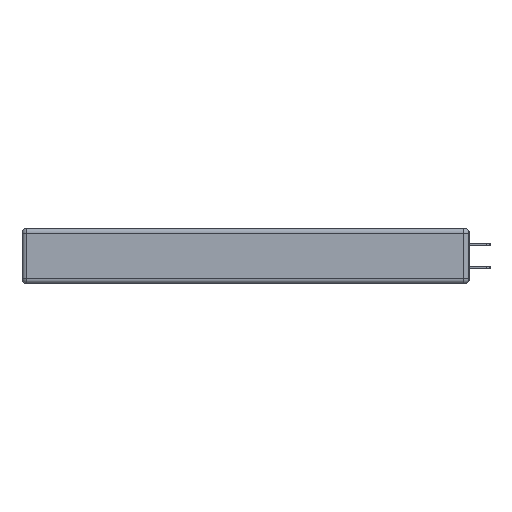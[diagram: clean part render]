
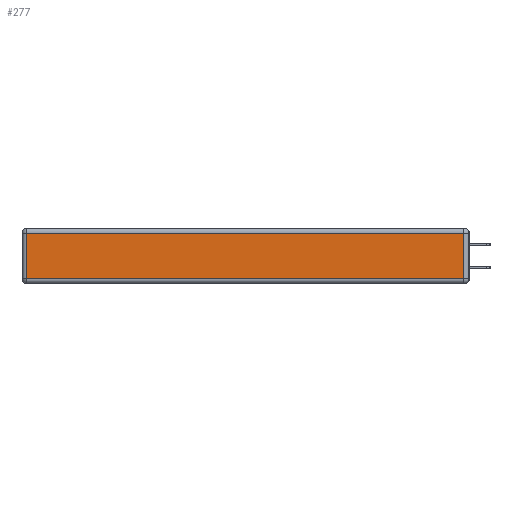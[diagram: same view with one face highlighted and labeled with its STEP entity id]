
A CAD part, left-side view. The second image highlights one B-rep face of the part: STEP entity #277.
In plain terms, the highlighted planar face has unit normal (-1, 0, 0).
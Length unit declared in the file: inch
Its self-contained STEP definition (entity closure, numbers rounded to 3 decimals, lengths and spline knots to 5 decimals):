
#159 = ORIENTED_EDGE ( 'NONE', *, *, #12862, .T. ) ;
#277 = ADVANCED_FACE ( 'NONE', ( #6587 ), #22933, .T. ) ;
#910 = CARTESIAN_POINT ( 'NONE',  ( 0., 0., -0.313 ) ) ;
#964 = VERTEX_POINT ( 'NONE', #26916 ) ;
#1173 = CARTESIAN_POINT ( 'NONE',  ( 0., 0.03, -0.313 ) ) ;
#3759 = DIRECTION ( 'NONE',  ( 0., 1., 0. ) ) ;
#4067 = DIRECTION ( 'NONE',  ( -1., 0., 0. ) ) ;
#4335 = DIRECTION ( 'NONE',  ( 0., 0., 1. ) ) ;
#6587 = FACE_OUTER_BOUND ( 'NONE', #15515, .T. ) ;
#6824 = ORIENTED_EDGE ( 'NONE', *, *, #15740, .T. ) ;
#7774 = LINE ( 'NONE', #7867, #15667 ) ;
#7867 = CARTESIAN_POINT ( 'NONE',  ( 0., 2.75, -0.03 ) ) ;
#8968 = CARTESIAN_POINT ( 'NONE',  ( 0., 2.72, -0.343 ) ) ;
#9300 = ORIENTED_EDGE ( 'NONE', *, *, #17796, .T. ) ;
#12862 = EDGE_CURVE ( 'NONE', #22538, #964, #18103, .T. ) ;
#14805 = CARTESIAN_POINT ( 'NONE',  ( 0., 0.03, -0.343 ) ) ;
#15221 = LINE ( 'NONE', #910, #18449 ) ;
#15515 = EDGE_LOOP ( 'NONE', ( #9300, #159, #6824, #23029 ) ) ;
#15667 = VECTOR ( 'NONE', #3759, 39.37008 ) ;
#15740 = EDGE_CURVE ( 'NONE', #964, #25596, #7774, .T. ) ;
#15995 = CARTESIAN_POINT ( 'NONE',  ( 0., 2.72, -0.03 ) ) ;
#17796 = EDGE_CURVE ( 'NONE', #23137, #22538, #15221, .T. ) ;
#18103 = LINE ( 'NONE', #14805, #22332 ) ;
#18449 = VECTOR ( 'NONE', #23837, 39.37008 ) ;
#18556 = CARTESIAN_POINT ( 'NONE',  ( 0., 0., -0.343 ) ) ;
#18739 = DIRECTION ( 'NONE',  ( 0., 0., 1. ) ) ;
#18831 = VECTOR ( 'NONE', #21544, 39.37008 ) ;
#21544 = DIRECTION ( 'NONE',  ( 0., 0., -1. ) ) ;
#22294 = CARTESIAN_POINT ( 'NONE',  ( 0., 2.72, -0.313 ) ) ;
#22332 = VECTOR ( 'NONE', #4335, 39.37008 ) ;
#22538 = VERTEX_POINT ( 'NONE', #1173 ) ;
#22933 = PLANE ( 'NONE',  #25558 ) ;
#23029 = ORIENTED_EDGE ( 'NONE', *, *, #25000, .T. ) ;
#23137 = VERTEX_POINT ( 'NONE', #22294 ) ;
#23714 = LINE ( 'NONE', #8968, #18831 ) ;
#23837 = DIRECTION ( 'NONE',  ( 0., -1., 0. ) ) ;
#25000 = EDGE_CURVE ( 'NONE', #25596, #23137, #23714, .T. ) ;
#25558 = AXIS2_PLACEMENT_3D ( 'NONE', #18556, #4067, #18739 ) ;
#25596 = VERTEX_POINT ( 'NONE', #15995 ) ;
#26916 = CARTESIAN_POINT ( 'NONE',  ( 0., 0.03, -0.03 ) ) ;
